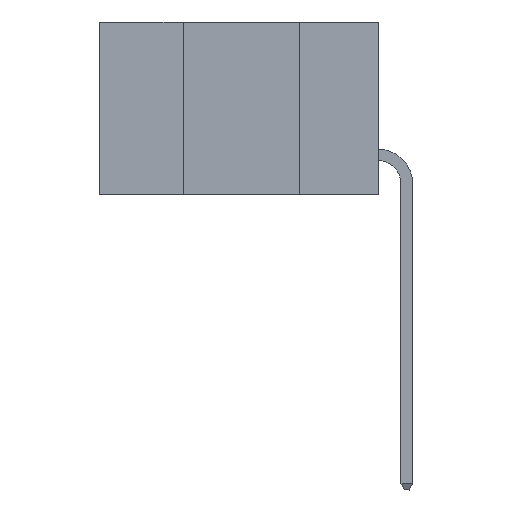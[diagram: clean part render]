
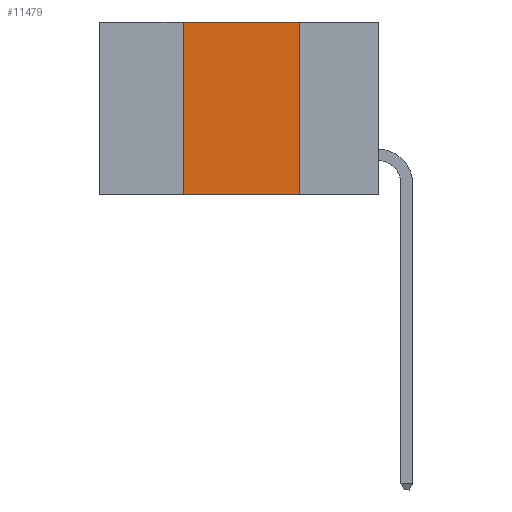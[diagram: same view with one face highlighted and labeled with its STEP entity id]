
A CAD part, left-side view. The second image highlights one B-rep face of the part: STEP entity #11479.
In plain terms, the highlighted planar face has unit normal (-1, 0, 0).
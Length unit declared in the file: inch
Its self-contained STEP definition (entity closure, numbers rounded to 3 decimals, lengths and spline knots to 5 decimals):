
#830 = CARTESIAN_POINT ( 'NONE',  ( 0., 0.6, -0.37 ) ) ;
#1332 = DIRECTION ( 'NONE',  ( 0., -1., 0. ) ) ;
#1722 = ORIENTED_EDGE ( 'NONE', *, *, #11987, .F. ) ;
#3625 = LINE ( 'NONE', #19795, #16820 ) ;
#3785 = LINE ( 'NONE', #11937, #19797 ) ;
#5058 = ORIENTED_EDGE ( 'NONE', *, *, #9168, .F. ) ;
#5471 = LINE ( 'NONE', #830, #25049 ) ;
#5733 = EDGE_LOOP ( 'NONE', ( #5058, #26230, #1722, #25128 ) ) ;
#6981 = AXIS2_PLACEMENT_3D ( 'NONE', #13575, #21737, #9850 ) ;
#7430 = PLANE ( 'NONE',  #6981 ) ;
#7710 = EDGE_CURVE ( 'NONE', #21691, #22272, #5471, .T. ) ;
#9168 = EDGE_CURVE ( 'NONE', #18769, #22272, #3625, .T. ) ;
#9850 = DIRECTION ( 'NONE',  ( 0., 0., -1. ) ) ;
#11479 = ADVANCED_FACE ( 'NONE', ( #25734 ), #7430, .F. ) ;
#11937 = CARTESIAN_POINT ( 'NONE',  ( 0., 0.42, -0.37 ) ) ;
#11987 = EDGE_CURVE ( 'NONE', #21691, #16818, #3785, .T. ) ;
#12544 = CARTESIAN_POINT ( 'NONE',  ( 0., 0.42, -0.37 ) ) ;
#13575 = CARTESIAN_POINT ( 'NONE',  ( 0., 0.6, 0. ) ) ;
#14279 = LINE ( 'NONE', #21816, #18820 ) ;
#15979 = CARTESIAN_POINT ( 'NONE',  ( 0., 0.17, -0.37 ) ) ;
#16818 = VERTEX_POINT ( 'NONE', #18753 ) ;
#16820 = VECTOR ( 'NONE', #24068, 39.37008 ) ;
#18753 = CARTESIAN_POINT ( 'NONE',  ( 0., 0.42, 0. ) ) ;
#18769 = VERTEX_POINT ( 'NONE', #25962 ) ;
#18820 = VECTOR ( 'NONE', #20166, 39.37008 ) ;
#19795 = CARTESIAN_POINT ( 'NONE',  ( 0., 0.17, -0.37 ) ) ;
#19797 = VECTOR ( 'NONE', #20347, 39.37008 ) ;
#20166 = DIRECTION ( 'NONE',  ( 0., -1., 0. ) ) ;
#20347 = DIRECTION ( 'NONE',  ( 0., 0., 1. ) ) ;
#21691 = VERTEX_POINT ( 'NONE', #12544 ) ;
#21737 = DIRECTION ( 'NONE',  ( 1., 0., 0. ) ) ;
#21816 = CARTESIAN_POINT ( 'NONE',  ( 0., 0.6, 0. ) ) ;
#21880 = EDGE_CURVE ( 'NONE', #16818, #18769, #14279, .T. ) ;
#22272 = VERTEX_POINT ( 'NONE', #15979 ) ;
#24068 = DIRECTION ( 'NONE',  ( 0., 0., -1. ) ) ;
#25049 = VECTOR ( 'NONE', #1332, 39.37008 ) ;
#25128 = ORIENTED_EDGE ( 'NONE', *, *, #7710, .T. ) ;
#25734 = FACE_OUTER_BOUND ( 'NONE', #5733, .T. ) ;
#25962 = CARTESIAN_POINT ( 'NONE',  ( 0., 0.17, 0. ) ) ;
#26230 = ORIENTED_EDGE ( 'NONE', *, *, #21880, .F. ) ;
